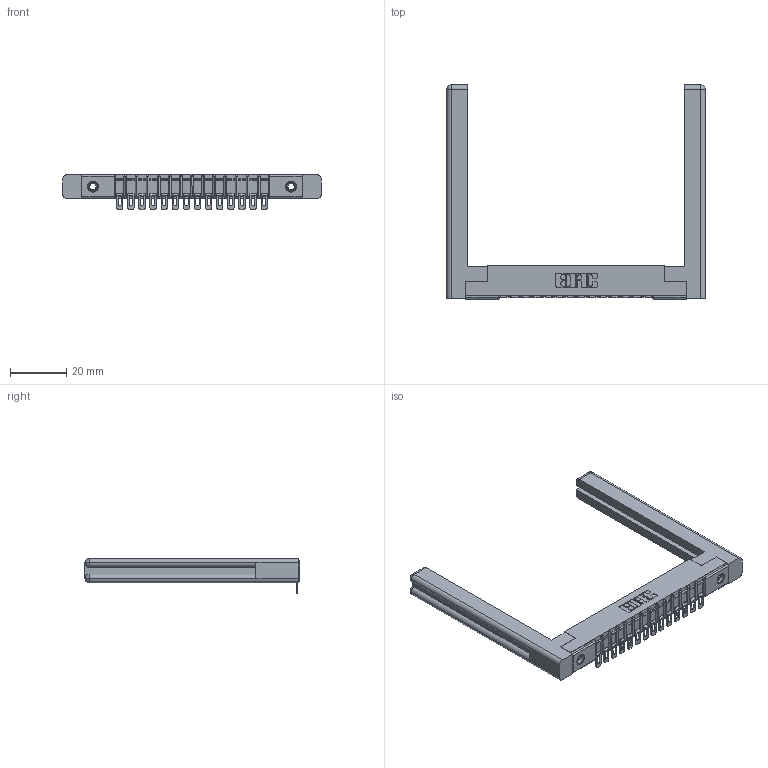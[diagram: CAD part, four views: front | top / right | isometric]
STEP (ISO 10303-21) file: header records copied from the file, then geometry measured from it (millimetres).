
FILE_DESCRIPTION (( 'STEP AP203' ), '1' );
FILE_NAME ('357-014-454-158.STEP', '2020-09-30T16:26:39', ( '' ), ( '' ), 'SwSTEP 2.0', 'SolidWorks 2020', '' );
FILE_SCHEMA (( 'CONFIG_CONTROL_DESIGN' ));
Length unit declared in the file: inch
Products named in the file (5): 307-220-058; 345-250-001_345-250-001-102; 307-290-002_554; 307 Part_.156 Dia Mounting Holes; 357-014-454-158
Assembly tree (19 placements, depth 2):
  357-014-454-158
    307 Part_.156 Dia Mounting Holes
    307-290-002_554  x14
    307-220-058  x2
    345-250-001_345-250-001-102  x2
Bounding box: 92.1 x 76.33 x 12.52 mm (x, y, z)
Volume: 13759.5 mm3; surface area: 15697.7 mm2
Topology: 19 solids, 19 shells, 1409 faces, 4219 edges, 2758 vertices
Faces by surface type: plane 798, cylinder 557, sphere 30, torus 12, cone 12
Entity records: 19052 total; most frequent: CARTESIAN_POINT 3217, ORIENTED_EDGE 3146, DIRECTION 3105, EDGE_CURVE 1573, VECTOR 1181, LINE 1181, VERTEX_POINT 1020, AXIS2_PLACEMENT_3D 962
